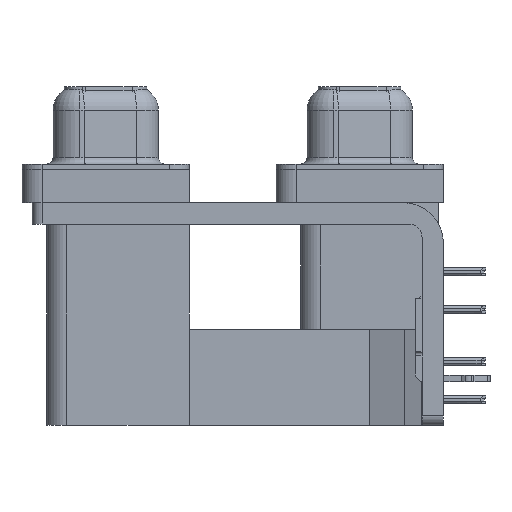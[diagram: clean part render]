
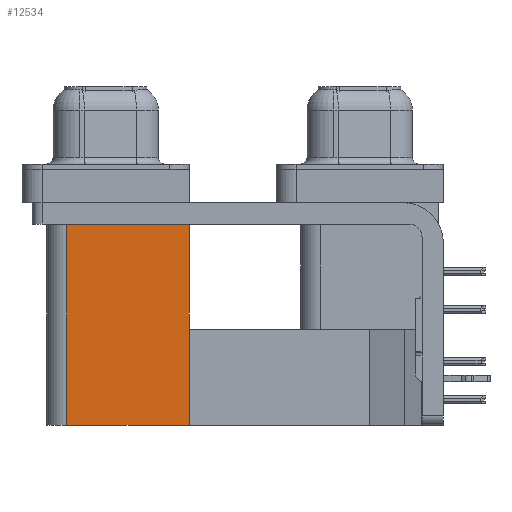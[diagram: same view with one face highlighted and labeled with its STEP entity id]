
A CAD part, left-side view. The second image highlights one B-rep face of the part: STEP entity #12534.
In plain terms, the highlighted planar face has unit normal (-1, 0, 0).
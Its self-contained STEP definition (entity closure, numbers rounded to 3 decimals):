
#2177 = EDGE_CURVE ( 'NONE', #22168, #34015, #23283, .T. ) ;
#2612 = CARTESIAN_POINT ( 'NONE',  ( 3.79, 21.975, -2.5 ) ) ;
#3239 = EDGE_CURVE ( 'NONE', #23740, #34015, #27957, .T. ) ;
#4477 = CARTESIAN_POINT ( 'NONE',  ( 3.79, 12.775, -19.2 ) ) ;
#4633 = CARTESIAN_POINT ( 'NONE',  ( 3.79, 12.775, -19.2 ) ) ;
#6623 = CARTESIAN_POINT ( 'NONE',  ( 3.79, 21.975, -19.2 ) ) ;
#7126 = LINE ( 'NONE', #14626, #14910 ) ;
#8159 = CARTESIAN_POINT ( 'NONE',  ( 3.79, 12.775, -2.5 ) ) ;
#9607 = DIRECTION ( 'NONE',  ( 1., 0., 0. ) ) ;
#10746 = ORIENTED_EDGE ( 'NONE', *, *, #37103, .T. ) ;
#11265 = DIRECTION ( 'NONE',  ( 0., 0., 1. ) ) ;
#11575 = VECTOR ( 'NONE', #35378, 1000. ) ;
#12534 = ADVANCED_FACE ( 'NONE', ( #19822 ), #40512, .F. ) ;
#13292 = DIRECTION ( 'NONE',  ( 0., 0., 1. ) ) ;
#14626 = CARTESIAN_POINT ( 'NONE',  ( 3.79, 12.775, -19.2 ) ) ;
#14910 = VECTOR ( 'NONE', #11265, 1000. ) ;
#17231 = ORIENTED_EDGE ( 'NONE', *, *, #2177, .F. ) ;
#18449 = EDGE_CURVE ( 'NONE', #42798, #22168, #29141, .T. ) ;
#19822 = FACE_OUTER_BOUND ( 'NONE', #33820, .T. ) ;
#20734 = VECTOR ( 'NONE', #13292, 1000. ) ;
#22168 = VERTEX_POINT ( 'NONE', #34573 ) ;
#23283 = LINE ( 'NONE', #6623, #20734 ) ;
#23553 = ORIENTED_EDGE ( 'NONE', *, *, #3239, .T. ) ;
#23740 = VERTEX_POINT ( 'NONE', #35792 ) ;
#26324 = ORIENTED_EDGE ( 'NONE', *, *, #18449, .F. ) ;
#27175 = DIRECTION ( 'NONE',  ( 0., 1., 0. ) ) ;
#27957 = LINE ( 'NONE', #8159, #30700 ) ;
#29141 = LINE ( 'NONE', #4477, #11575 ) ;
#29820 = CARTESIAN_POINT ( 'NONE',  ( 3.79, 12.775, -19.2 ) ) ;
#30700 = VECTOR ( 'NONE', #31069, 1000. ) ;
#31069 = DIRECTION ( 'NONE',  ( 0., 1., 0. ) ) ;
#33464 = AXIS2_PLACEMENT_3D ( 'NONE', #29820, #9607, #27175 ) ;
#33820 = EDGE_LOOP ( 'NONE', ( #23553, #17231, #26324, #10746 ) ) ;
#34015 = VERTEX_POINT ( 'NONE', #2612 ) ;
#34573 = CARTESIAN_POINT ( 'NONE',  ( 3.79, 21.975, -19.2 ) ) ;
#35378 = DIRECTION ( 'NONE',  ( 0., 1., 0. ) ) ;
#35792 = CARTESIAN_POINT ( 'NONE',  ( 3.79, 12.775, -2.5 ) ) ;
#37103 = EDGE_CURVE ( 'NONE', #42798, #23740, #7126, .T. ) ;
#40512 = PLANE ( 'NONE',  #33464 ) ;
#42798 = VERTEX_POINT ( 'NONE', #4633 ) ;
